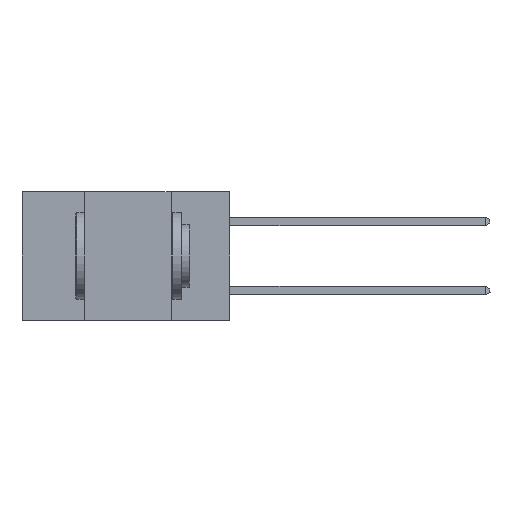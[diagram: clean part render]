
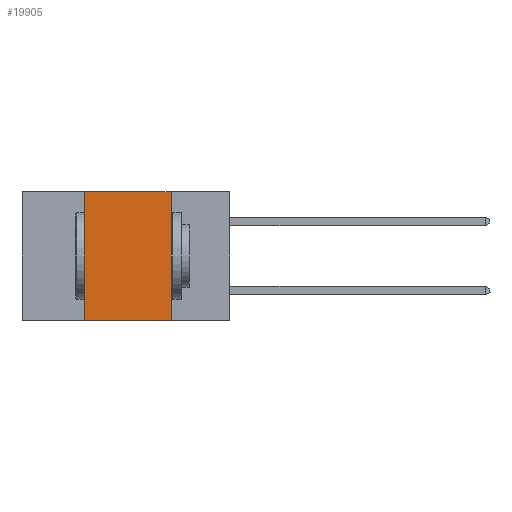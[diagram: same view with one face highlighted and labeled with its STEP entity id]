
A CAD part, left-side view. The second image highlights one B-rep face of the part: STEP entity #19905.
In plain terms, the highlighted planar face has unit normal (-1, 0, 0).
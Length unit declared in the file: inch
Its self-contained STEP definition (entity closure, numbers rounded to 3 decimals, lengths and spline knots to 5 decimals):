
#495 = DIRECTION ( 'NONE',  ( 0., 0., -1. ) ) ;
#736 = DIRECTION ( 'NONE',  ( 0., -1., 0. ) ) ;
#788 = ORIENTED_EDGE ( 'NONE', *, *, #16269, .F. ) ;
#847 = AXIS2_PLACEMENT_3D ( 'NONE', #6129, #7753, #4611 ) ;
#1490 = EDGE_CURVE ( 'NONE', #6987, #16022, #1569, .T. ) ;
#1569 = LINE ( 'NONE', #13575, #18231 ) ;
#1714 = ORIENTED_EDGE ( 'NONE', *, *, #1490, .F. ) ;
#2430 = ORIENTED_EDGE ( 'NONE', *, *, #12626, .T. ) ;
#2473 = VECTOR ( 'NONE', #3153, 39.37008 ) ;
#3153 = DIRECTION ( 'NONE',  ( 0., -1., 0. ) ) ;
#4611 = DIRECTION ( 'NONE',  ( 0., 0., -1. ) ) ;
#4980 = VECTOR ( 'NONE', #20710, 39.37008 ) ;
#5792 = CARTESIAN_POINT ( 'NONE',  ( 0., 0.6, 0. ) ) ;
#5855 = CARTESIAN_POINT ( 'NONE',  ( 0., 0.42, -0.37 ) ) ;
#6129 = CARTESIAN_POINT ( 'NONE',  ( 0., 0.6, 0. ) ) ;
#6987 = VERTEX_POINT ( 'NONE', #10734 ) ;
#7753 = DIRECTION ( 'NONE',  ( 1., 0., 0. ) ) ;
#7825 = EDGE_LOOP ( 'NONE', ( #1714, #9709, #788, #2430 ) ) ;
#8321 = LINE ( 'NONE', #12715, #2473 ) ;
#9515 = CARTESIAN_POINT ( 'NONE',  ( 0., 0.42, 0. ) ) ;
#9709 = ORIENTED_EDGE ( 'NONE', *, *, #19044, .F. ) ;
#10716 = CARTESIAN_POINT ( 'NONE',  ( 0., 0.17, -0.37 ) ) ;
#10734 = CARTESIAN_POINT ( 'NONE',  ( 0., 0.17, 0. ) ) ;
#12626 = EDGE_CURVE ( 'NONE', #14188, #16022, #8321, .T. ) ;
#12715 = CARTESIAN_POINT ( 'NONE',  ( 0., 0.6, -0.37 ) ) ;
#13389 = FACE_OUTER_BOUND ( 'NONE', #7825, .T. ) ;
#13575 = CARTESIAN_POINT ( 'NONE',  ( 0., 0.17, 0. ) ) ;
#13698 = PLANE ( 'NONE',  #847 ) ;
#14188 = VERTEX_POINT ( 'NONE', #5855 ) ;
#14750 = VERTEX_POINT ( 'NONE', #15151 ) ;
#15151 = CARTESIAN_POINT ( 'NONE',  ( 0., 0.42, 0. ) ) ;
#16022 = VERTEX_POINT ( 'NONE', #10716 ) ;
#16269 = EDGE_CURVE ( 'NONE', #14188, #14750, #17837, .T. ) ;
#17837 = LINE ( 'NONE', #9515, #4980 ) ;
#18231 = VECTOR ( 'NONE', #495, 39.37008 ) ;
#19044 = EDGE_CURVE ( 'NONE', #14750, #6987, #19484, .T. ) ;
#19484 = LINE ( 'NONE', #5792, #19977 ) ;
#19905 = ADVANCED_FACE ( 'NONE', ( #13389 ), #13698, .F. ) ;
#19977 = VECTOR ( 'NONE', #736, 39.37008 ) ;
#20710 = DIRECTION ( 'NONE',  ( 0., 0., 1. ) ) ;
